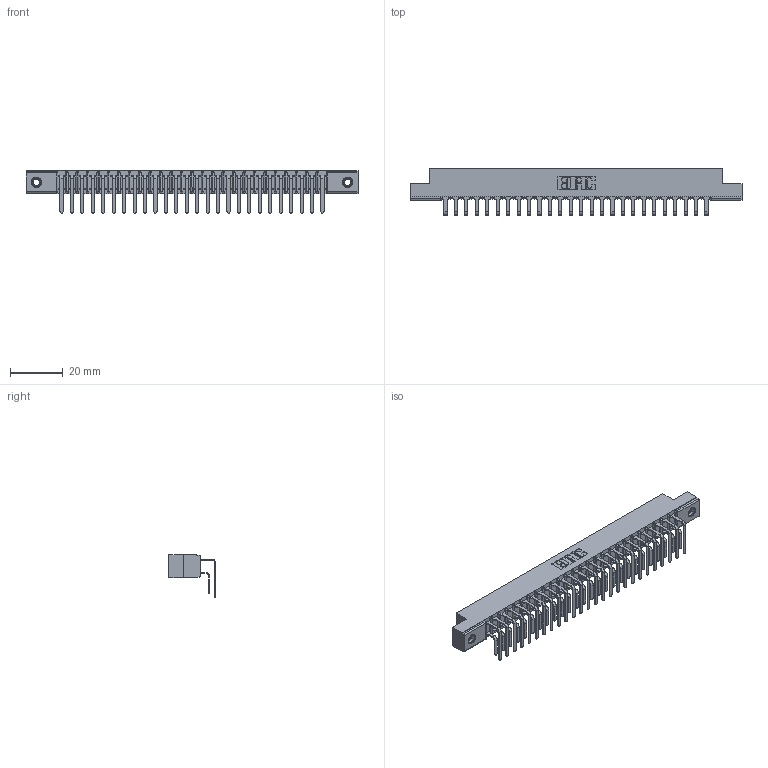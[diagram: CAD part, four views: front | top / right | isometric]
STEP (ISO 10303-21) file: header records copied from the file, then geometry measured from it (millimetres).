
FILE_DESCRIPTION (( 'STEP AP203' ), '1' );
FILE_NAME ('307-052-459-207.STEP', '2020-09-30T07:56:10', ( '' ), ( '' ), 'SwSTEP 2.0', 'SolidWorks 2020', '' );
FILE_SCHEMA (( 'CONFIG_CONTROL_DESIGN' ));
Length unit declared in the file: inch
Products named in the file (5): 307-290-001_559 - 2 (Single); 307 Part_.156 Dia Mounting Holes; 307-052-459-207; 345-250-001_345-250-005-103; 307-290-001_558 559 - 1 (Single)
Assembly tree (55 placements, depth 2):
  307-052-459-207
    307 Part_.156 Dia Mounting Holes
    307-290-001_558 559 - 1 (Single)  x26
    307-290-001_559 - 2 (Single)  x26
    345-250-001_345-250-005-103  x2
Bounding box: 126.03 x 17.69 x 16.08 mm (x, y, z)
Volume: 8460.6 mm3; surface area: 16487.9 mm2
Topology: 55 solids, 55 shells, 2805 faces, 7843 edges, 5078 vertices
Faces by surface type: plane 1818, cylinder 917, sphere 54, cone 12, torus 4
Entity records: 27726 total; most frequent: CARTESIAN_POINT 4527, ORIENTED_EDGE 4478, DIRECTION 4449, EDGE_CURVE 2239, LINE 1709, VECTOR 1709, VERTEX_POINT 1448, AXIS2_PLACEMENT_3D 1370
